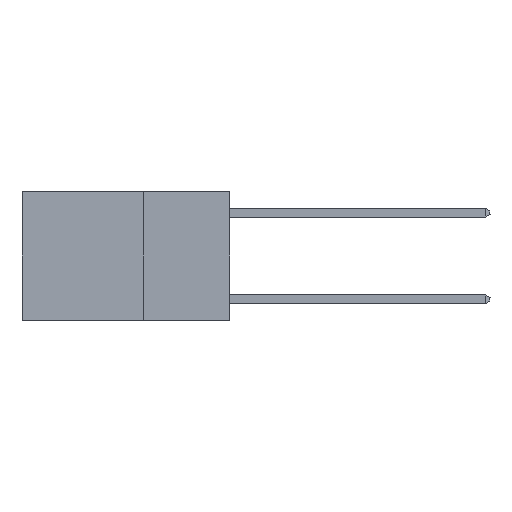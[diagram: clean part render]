
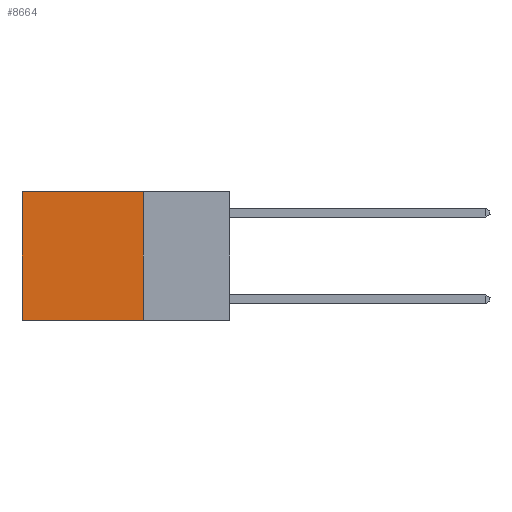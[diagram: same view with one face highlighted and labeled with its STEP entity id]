
A CAD part, left-side view. The second image highlights one B-rep face of the part: STEP entity #8664.
In plain terms, the highlighted planar face has unit normal (-1, 0, 0).
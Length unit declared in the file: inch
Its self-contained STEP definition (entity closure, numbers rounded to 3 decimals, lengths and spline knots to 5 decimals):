
#1164 = VECTOR ( 'NONE', #15610, 39.37008 ) ;
#1210 = VERTEX_POINT ( 'NONE', #8378 ) ;
#1392 = DIRECTION ( 'NONE',  ( 0., 0., -1. ) ) ;
#1494 = EDGE_CURVE ( 'NONE', #19041, #10814, #19241, .T. ) ;
#3569 = CARTESIAN_POINT ( 'NONE',  ( 0.2625, 0.6, 0. ) ) ;
#3611 = DIRECTION ( 'NONE',  ( 0., 0., -1. ) ) ;
#5199 = EDGE_CURVE ( 'NONE', #10321, #1210, #19206, .T. ) ;
#7457 = VECTOR ( 'NONE', #1392, 39.37008 ) ;
#7589 = AXIS2_PLACEMENT_3D ( 'NONE', #22350, #16001, #22112 ) ;
#7791 = LINE ( 'NONE', #15873, #1164 ) ;
#8378 = CARTESIAN_POINT ( 'NONE',  ( 0.2625, 0.6, -0.37 ) ) ;
#8664 = ADVANCED_FACE ( 'NONE', ( #20191 ), #14436, .F. ) ;
#9337 = CARTESIAN_POINT ( 'NONE',  ( 0.2625, 0.6, 0. ) ) ;
#10321 = VERTEX_POINT ( 'NONE', #9337 ) ;
#10814 = VERTEX_POINT ( 'NONE', #23596 ) ;
#11484 = ORIENTED_EDGE ( 'NONE', *, *, #21854, .F. ) ;
#11899 = DIRECTION ( 'NONE',  ( 0., 1., 0. ) ) ;
#11902 = EDGE_CURVE ( 'NONE', #19041, #10321, #12019, .T. ) ;
#12019 = LINE ( 'NONE', #15842, #22678 ) ;
#14425 = VECTOR ( 'NONE', #3611, 39.37008 ) ;
#14436 = PLANE ( 'NONE',  #7589 ) ;
#15610 = DIRECTION ( 'NONE',  ( 0., 1., 0. ) ) ;
#15842 = CARTESIAN_POINT ( 'NONE',  ( 0.2625, 0.25, 0. ) ) ;
#15873 = CARTESIAN_POINT ( 'NONE',  ( 0.2625, 0.25, -0.37 ) ) ;
#16001 = DIRECTION ( 'NONE',  ( 1., 0., 0. ) ) ;
#17704 = CARTESIAN_POINT ( 'NONE',  ( 0.2625, 0.25, 0. ) ) ;
#19041 = VERTEX_POINT ( 'NONE', #20135 ) ;
#19206 = LINE ( 'NONE', #3569, #7457 ) ;
#19241 = LINE ( 'NONE', #17704, #14425 ) ;
#20135 = CARTESIAN_POINT ( 'NONE',  ( 0.2625, 0.25, 0. ) ) ;
#20191 = FACE_OUTER_BOUND ( 'NONE', #24058, .T. ) ;
#21854 = EDGE_CURVE ( 'NONE', #10814, #1210, #7791, .T. ) ;
#22112 = DIRECTION ( 'NONE',  ( 0., 0., -1. ) ) ;
#22350 = CARTESIAN_POINT ( 'NONE',  ( 0.2625, 0.25, 0. ) ) ;
#22433 = ORIENTED_EDGE ( 'NONE', *, *, #5199, .T. ) ;
#22678 = VECTOR ( 'NONE', #11899, 39.37008 ) ;
#22954 = ORIENTED_EDGE ( 'NONE', *, *, #1494, .F. ) ;
#23596 = CARTESIAN_POINT ( 'NONE',  ( 0.2625, 0.25, -0.37 ) ) ;
#24058 = EDGE_LOOP ( 'NONE', ( #22433, #11484, #22954, #24713 ) ) ;
#24713 = ORIENTED_EDGE ( 'NONE', *, *, #11902, .T. ) ;
